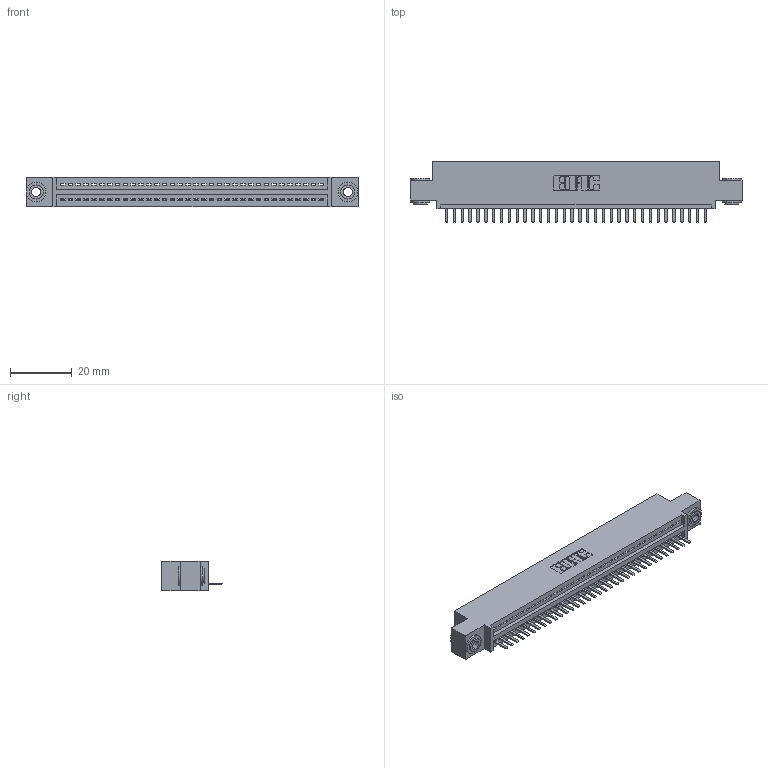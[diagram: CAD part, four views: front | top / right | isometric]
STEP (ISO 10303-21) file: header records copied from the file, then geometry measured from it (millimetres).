
FILE_DESCRIPTION (( 'STEP AP203' ), '1' );
FILE_NAME ('345-034-520-403.STEP', '2018-08-29T00:02:08', ( '' ), ( '' ), 'SwSTEP 2.0', 'SolidWorks 2016', '' );
FILE_SCHEMA (( 'CONFIG_CONTROL_DESIGN' ));
Length unit declared in the file: inch
Products named in the file (4): 345 Part_0.110 Offset - 0.156 Dia-TH; 345-292-001_345-293-120; 345-250-002_345-250-002-102; 345-034-520-403
Assembly tree (37 placements, depth 2):
  345-034-520-403
    345 Part_0.110 Offset - 0.156 Dia-TH
    345-292-001_345-293-120  x34
    345-250-002_345-250-002-102  x2
Bounding box: 107.57 x 19.68 x 9.4 mm (x, y, z)
Volume: 9999.7 mm3; surface area: 13156.4 mm2
Topology: 37 solids, 37 shells, 2276 faces, 6685 edges, 4362 vertices
Faces by surface type: plane 1522, cylinder 746, cone 8
Entity records: 27562 total; most frequent: CARTESIAN_POINT 4765, ORIENTED_EDGE 4714, DIRECTION 4191, EDGE_CURVE 2357, LINE 2061, VECTOR 2061, VERTEX_POINT 1566, AXIS2_PLACEMENT_3D 1065
